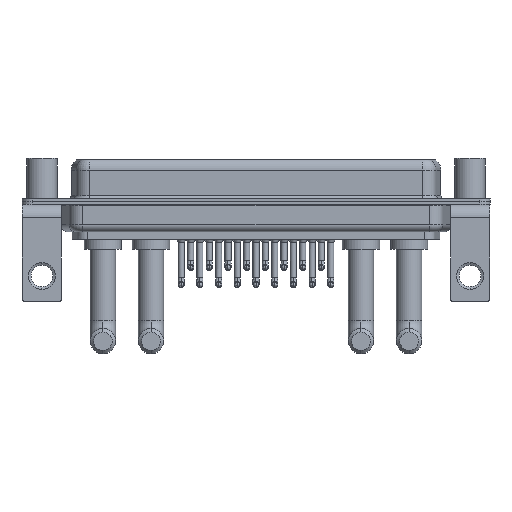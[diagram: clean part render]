
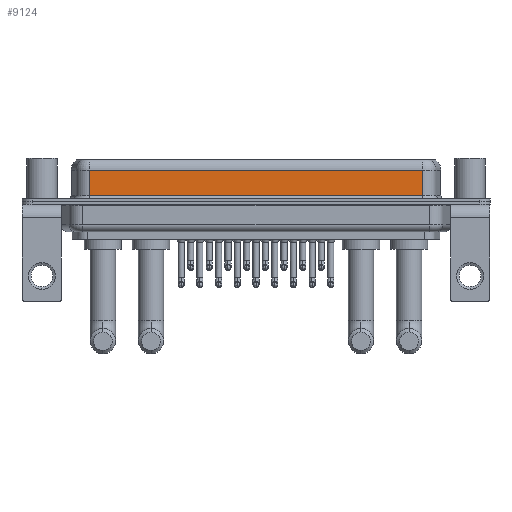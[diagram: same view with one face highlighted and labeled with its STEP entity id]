
A CAD part, front view. The second image highlights one B-rep face of the part: STEP entity #9124.
In plain terms, the highlighted planar face has unit normal (0, -1, 0).
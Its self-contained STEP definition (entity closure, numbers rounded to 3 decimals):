
#103 = LINE ( 'NONE', #4218, #6545 ) ;
#2326 = CARTESIAN_POINT ( 'NONE',  ( 56.462, -3.95, 4.65 ) ) ;
#3628 = ORIENTED_EDGE ( 'NONE', *, *, #4115, .T. ) ;
#3766 = VECTOR ( 'NONE', #6618, 1000. ) ;
#4059 = CARTESIAN_POINT ( 'NONE',  ( 7.038, -3.95, 4.65 ) ) ;
#4115 = EDGE_CURVE ( 'NONE', #4712, #15857, #103, .T. ) ;
#4218 = CARTESIAN_POINT ( 'NONE',  ( 7.038, -3.95, 6.4 ) ) ;
#4312 = DIRECTION ( 'NONE',  ( 0., 1., 0. ) ) ;
#4604 = CARTESIAN_POINT ( 'NONE',  ( 7.038, -3.95, 0.9 ) ) ;
#4712 = VERTEX_POINT ( 'NONE', #4059 ) ;
#4851 = CARTESIAN_POINT ( 'NONE',  ( 56.462, -3.95, 6.4 ) ) ;
#5892 = EDGE_CURVE ( 'NONE', #15857, #11816, #14090, .T. ) ;
#6545 = VECTOR ( 'NONE', #21365, 1000. ) ;
#6618 = DIRECTION ( 'NONE',  ( 1., 0., 0. ) ) ;
#7190 = EDGE_CURVE ( 'NONE', #23646, #11816, #12343, .T. ) ;
#9124 = ADVANCED_FACE ( 'NONE', ( #17769 ), #20965, .F. ) ;
#9940 = CARTESIAN_POINT ( 'NONE',  ( 56.462, -3.95, 6.4 ) ) ;
#9982 = CARTESIAN_POINT ( 'NONE',  ( 56.462, -3.95, 0.9 ) ) ;
#11055 = EDGE_LOOP ( 'NONE', ( #17583, #16771, #3628, #22540 ) ) ;
#11816 = VERTEX_POINT ( 'NONE', #9982 ) ;
#12343 = LINE ( 'NONE', #4851, #22086 ) ;
#12935 = LINE ( 'NONE', #15021, #18272 ) ;
#14090 = LINE ( 'NONE', #17827, #3766 ) ;
#15021 = CARTESIAN_POINT ( 'NONE',  ( 56.462, -3.95, 4.65 ) ) ;
#15140 = DIRECTION ( 'NONE',  ( -1., 0., 0. ) ) ;
#15857 = VERTEX_POINT ( 'NONE', #4604 ) ;
#16567 = DIRECTION ( 'NONE',  ( 0., 0., -1. ) ) ;
#16771 = ORIENTED_EDGE ( 'NONE', *, *, #19745, .T. ) ;
#17583 = ORIENTED_EDGE ( 'NONE', *, *, #7190, .F. ) ;
#17769 = FACE_OUTER_BOUND ( 'NONE', #11055, .T. ) ;
#17827 = CARTESIAN_POINT ( 'NONE',  ( 56.462, -3.95, 0.9 ) ) ;
#18272 = VECTOR ( 'NONE', #15140, 1000. ) ;
#18587 = AXIS2_PLACEMENT_3D ( 'NONE', #9940, #4312, #19611 ) ;
#19611 = DIRECTION ( 'NONE',  ( 0., 0., 1. ) ) ;
#19745 = EDGE_CURVE ( 'NONE', #23646, #4712, #12935, .T. ) ;
#20965 = PLANE ( 'NONE',  #18587 ) ;
#21365 = DIRECTION ( 'NONE',  ( 0., 0., -1. ) ) ;
#22086 = VECTOR ( 'NONE', #16567, 1000. ) ;
#22540 = ORIENTED_EDGE ( 'NONE', *, *, #5892, .T. ) ;
#23646 = VERTEX_POINT ( 'NONE', #2326 ) ;
